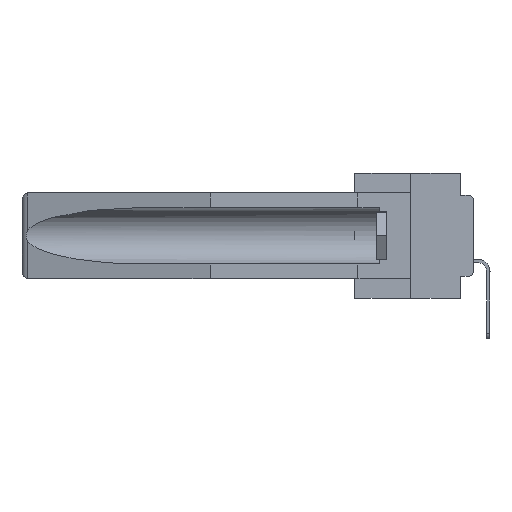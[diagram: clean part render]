
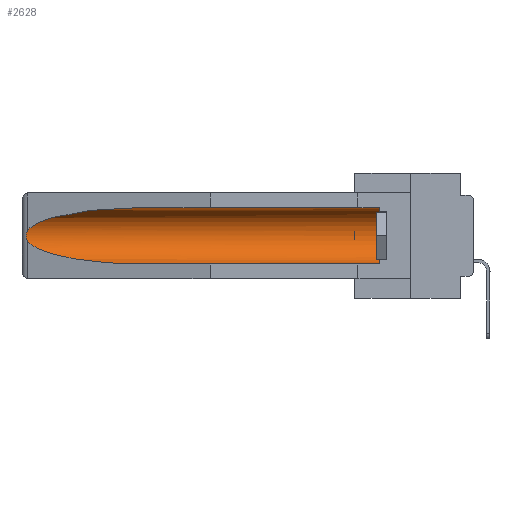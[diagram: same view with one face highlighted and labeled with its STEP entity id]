
A CAD part, left-side view. The second image highlights one B-rep face of the part: STEP entity #2628.
In plain terms, the highlighted cylindrical face has radius 2.857 mm (diameter 5.715 mm), a partial arc.
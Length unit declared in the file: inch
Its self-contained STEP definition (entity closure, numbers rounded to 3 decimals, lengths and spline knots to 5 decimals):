
#896 = ORIENTED_EDGE ( 'NONE', *, *, #4281, .T. ) ;
#1906 = CARTESIAN_POINT ( 'NONE',  ( 0.25451, 1.48313, -0.09465 ) ) ;
#1990 = ORIENTED_EDGE ( 'NONE', *, *, #38972, .F. ) ;
#2352 = B_SPLINE_CURVE_WITH_KNOTS ( 'NONE', 3,
 ( #7979, #38770, #33099, #11022, #11221, #20336, #29658, #35549, #23374, #38962 ),
 .UNSPECIFIED., .F., .F.,
 ( 4, 2, 2, 2, 4 ),
 ( 0., 0.00029, 0.00058, 0.00087, 0.00117 ),
 .UNSPECIFIED. ) ;
#2628 = ADVANCED_FACE ( 'NONE', ( #35020 ), #35427, .F. ) ;
#3111 = CARTESIAN_POINT ( 'NONE',  ( 0.155, 1.07973, -0.059 ) ) ;
#3234 = VECTOR ( 'NONE', #35045, 39.37008 ) ;
#3454 = DIRECTION ( 'NONE',  ( 0., -1., 0. ) ) ;
#4281 = EDGE_CURVE ( 'NONE', #8842, #33231, #9947, .T. ) ;
#5211 = DIRECTION ( 'NONE',  ( 0., 1., 0. ) ) ;
#7979 = CARTESIAN_POINT ( 'NONE',  ( 0.26537, 1.52718, -0.14972 ) ) ;
#8074 = CARTESIAN_POINT ( 'NONE',  ( 0.155, -0.30754, -0.1715 ) ) ;
#8842 = VERTEX_POINT ( 'NONE', #3111 ) ;
#9837 = VERTEX_POINT ( 'NONE', #25691 ) ;
#9947 =( BOUNDED_CURVE ( )  B_SPLINE_CURVE ( 3, ( #29675, #15082, #1906, #18110 ),
 .UNSPECIFIED., .F., .T. ) 
 B_SPLINE_CURVE_WITH_KNOTS ( ( 4, 4 ),
 ( 4.71239, 6.08839 ),
 .UNSPECIFIED. ) 
 CURVE ( )  GEOMETRIC_REPRESENTATION_ITEM ( )  RATIONAL_B_SPLINE_CURVE ( ( 1., 0.848, 0.848, 1. ) ) 
 REPRESENTATION_ITEM ( '' )  );
#11022 = CARTESIAN_POINT ( 'NONE',  ( 0.2673, 1.5327, -0.16383 ) ) ;
#11221 = CARTESIAN_POINT ( 'NONE',  ( 0.2675, 1.53308, -0.16763 ) ) ;
#12145 = LINE ( 'NONE', #20849, #31945 ) ;
#15082 = CARTESIAN_POINT ( 'NONE',  ( 0.21114, 1.30732, -0.059 ) ) ;
#15857 = EDGE_LOOP ( 'NONE', ( #896, #16068, #24695, #1990, #26179, #27148 ) ) ;
#16068 = ORIENTED_EDGE ( 'NONE', *, *, #32356, .T. ) ;
#16976 = CARTESIAN_POINT ( 'NONE',  ( 0.155, 0.126, -0.284 ) ) ;
#18015 = DIRECTION ( 'NONE',  ( 0., 1., 0. ) ) ;
#18110 = CARTESIAN_POINT ( 'NONE',  ( 0.26537, 1.52718, -0.14972 ) ) ;
#18314 = CIRCLE ( 'NONE', #29877, 0.1125 ) ;
#18747 = CARTESIAN_POINT ( 'NONE',  ( 0.26537, 1.52718, -0.19328 ) ) ;
#18852 = DIRECTION ( 'NONE',  ( 0., 0., 1. ) ) ;
#19622 = VERTEX_POINT ( 'NONE', #27020 ) ;
#20236 = AXIS2_PLACEMENT_3D ( 'NONE', #8074, #5211, #23867 ) ;
#20336 = CARTESIAN_POINT ( 'NONE',  ( 0.2675, 1.53308, -0.17534 ) ) ;
#20849 = CARTESIAN_POINT ( 'NONE',  ( 0.155, -0.30754, -0.284 ) ) ;
#21427 = EDGE_CURVE ( 'NONE', #28424, #19622, #18314, .T. ) ;
#23374 = CARTESIAN_POINT ( 'NONE',  ( 0.26597, 1.5296, -0.19026 ) ) ;
#23867 = DIRECTION ( 'NONE',  ( 0., 0., 1. ) ) ;
#24695 = ORIENTED_EDGE ( 'NONE', *, *, #36687, .T. ) ;
#25691 = CARTESIAN_POINT ( 'NONE',  ( 0.155, 1.07973, -0.284 ) ) ;
#26179 = ORIENTED_EDGE ( 'NONE', *, *, #21427, .T. ) ;
#27020 = CARTESIAN_POINT ( 'NONE',  ( 0.155, 0.126, -0.059 ) ) ;
#27148 = ORIENTED_EDGE ( 'NONE', *, *, #34288, .T. ) ;
#28424 = VERTEX_POINT ( 'NONE', #16976 ) ;
#28969 = CARTESIAN_POINT ( 'NONE',  ( 0.26537, 1.52718, -0.14972 ) ) ;
#29658 = CARTESIAN_POINT ( 'NONE',  ( 0.2673, 1.53269, -0.17917 ) ) ;
#29675 = CARTESIAN_POINT ( 'NONE',  ( 0.155, 1.07973, -0.059 ) ) ;
#29877 = AXIS2_PLACEMENT_3D ( 'NONE', #37096, #3454, #18852 ) ;
#31111 = CARTESIAN_POINT ( 'NONE',  ( 0.25451, 1.48313, -0.24835 ) ) ;
#31218 = CARTESIAN_POINT ( 'NONE',  ( 0.155, -0.30754, -0.059 ) ) ;
#31945 = VECTOR ( 'NONE', #18015, 39.37008 ) ;
#32356 = EDGE_CURVE ( 'NONE', #33231, #38573, #2352, .T. ) ;
#32421 =( BOUNDED_CURVE ( )  B_SPLINE_CURVE ( 3, ( #18747, #31111, #36380, #36978 ),
 .UNSPECIFIED., .F., .F. ) 
 B_SPLINE_CURVE_WITH_KNOTS ( ( 4, 4 ),
 ( 0.1948, 1.5708 ),
 .UNSPECIFIED. ) 
 CURVE ( )  GEOMETRIC_REPRESENTATION_ITEM ( )  RATIONAL_B_SPLINE_CURVE ( ( 1., 0.848, 0.848, 1. ) ) 
 REPRESENTATION_ITEM ( '' )  );
#33099 = CARTESIAN_POINT ( 'NONE',  ( 0.26654, 1.53092, -0.15636 ) ) ;
#33231 = VERTEX_POINT ( 'NONE', #28969 ) ;
#33659 = CARTESIAN_POINT ( 'NONE',  ( 0.26537, 1.52718, -0.19328 ) ) ;
#34288 = EDGE_CURVE ( 'NONE', #19622, #8842, #38080, .T. ) ;
#35020 = FACE_OUTER_BOUND ( 'NONE', #15857, .T. ) ;
#35045 = DIRECTION ( 'NONE',  ( 0., 1., 0. ) ) ;
#35427 = CYLINDRICAL_SURFACE ( 'NONE', #20236, 0.1125 ) ;
#35549 = CARTESIAN_POINT ( 'NONE',  ( 0.26655, 1.53094, -0.18657 ) ) ;
#36380 = CARTESIAN_POINT ( 'NONE',  ( 0.21114, 1.30732, -0.284 ) ) ;
#36687 = EDGE_CURVE ( 'NONE', #38573, #9837, #32421, .T. ) ;
#36978 = CARTESIAN_POINT ( 'NONE',  ( 0.155, 1.07973, -0.284 ) ) ;
#37096 = CARTESIAN_POINT ( 'NONE',  ( 0.155, 0.126, -0.1715 ) ) ;
#38080 = LINE ( 'NONE', #31218, #3234 ) ;
#38573 = VERTEX_POINT ( 'NONE', #33659 ) ;
#38770 = CARTESIAN_POINT ( 'NONE',  ( 0.26597, 1.52961, -0.15275 ) ) ;
#38962 = CARTESIAN_POINT ( 'NONE',  ( 0.26537, 1.52718, -0.19328 ) ) ;
#38972 = EDGE_CURVE ( 'NONE', #28424, #9837, #12145, .T. ) ;
